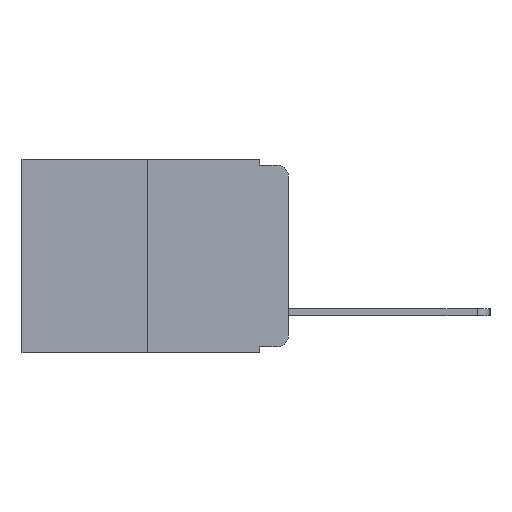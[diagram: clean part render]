
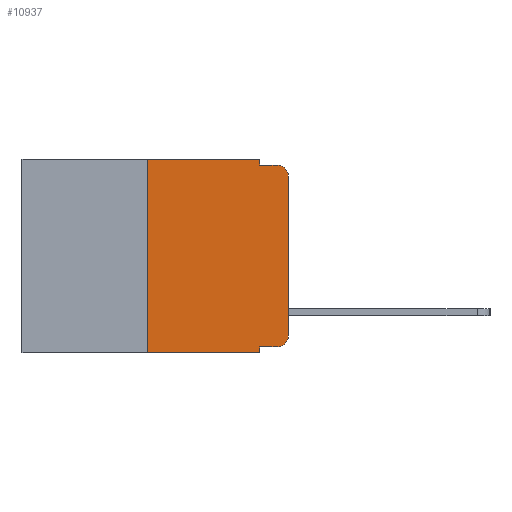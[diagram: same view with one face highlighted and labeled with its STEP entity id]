
A CAD part, left-side view. The second image highlights one B-rep face of the part: STEP entity #10937.
In plain terms, the highlighted planar face has unit normal (-1, 0, 0).
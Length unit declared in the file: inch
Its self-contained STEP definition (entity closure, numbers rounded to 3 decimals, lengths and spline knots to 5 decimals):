
#83 = EDGE_CURVE ( 'NONE', #4789, #15447, #14954, .T. ) ;
#96 = LINE ( 'NONE', #16927, #8019 ) ;
#361 = ORIENTED_EDGE ( 'NONE', *, *, #83, .F. ) ;
#401 = CARTESIAN_POINT ( 'NONE',  ( 0., 0.25, 0. ) ) ;
#1118 = ORIENTED_EDGE ( 'NONE', *, *, #17320, .T. ) ;
#1808 = LINE ( 'NONE', #2811, #13620 ) ;
#1845 = VECTOR ( 'NONE', #5247, 39.37008 ) ;
#2014 = DIRECTION ( 'NONE',  ( 0., 0., -1. ) ) ;
#2174 = VERTEX_POINT ( 'NONE', #8511 ) ;
#2244 = CARTESIAN_POINT ( 'NONE',  ( 0., 0.051, 0. ) ) ;
#2385 = EDGE_CURVE ( 'NONE', #12834, #7028, #96, .T. ) ;
#2429 = CIRCLE ( 'NONE', #7947, 0.02 ) ;
#2731 = DIRECTION ( 'NONE',  ( 0., 0., 1. ) ) ;
#2811 = CARTESIAN_POINT ( 'NONE',  ( 0., 0.051, 0. ) ) ;
#3052 = AXIS2_PLACEMENT_3D ( 'NONE', #17057, #8124, #18480 ) ;
#3173 = VECTOR ( 'NONE', #15278, 39.37008 ) ;
#3271 = EDGE_CURVE ( 'NONE', #6931, #4019, #18633, .T. ) ;
#3538 = VECTOR ( 'NONE', #13511, 39.37008 ) ;
#3826 = CARTESIAN_POINT ( 'NONE',  ( 0., 0.473, 0. ) ) ;
#4019 = VERTEX_POINT ( 'NONE', #2244 ) ;
#4202 = ORIENTED_EDGE ( 'NONE', *, *, #7983, .T. ) ;
#4789 = VERTEX_POINT ( 'NONE', #7397 ) ;
#5091 = FACE_OUTER_BOUND ( 'NONE', #15024, .T. ) ;
#5247 = DIRECTION ( 'NONE',  ( 0., -1., 0. ) ) ;
#5254 = DIRECTION ( 'NONE',  ( 0., 0., 1. ) ) ;
#5626 = ORIENTED_EDGE ( 'NONE', *, *, #8613, .T. ) ;
#6355 = ORIENTED_EDGE ( 'NONE', *, *, #9268, .F. ) ;
#6802 = VECTOR ( 'NONE', #17627, 39.37008 ) ;
#6863 = EDGE_CURVE ( 'NONE', #16658, #6931, #12802, .T. ) ;
#6915 = VECTOR ( 'NONE', #2014, 39.37008 ) ;
#6924 = DIRECTION ( 'NONE',  ( 1., 0., 0. ) ) ;
#6931 = VERTEX_POINT ( 'NONE', #8373 ) ;
#7028 = VERTEX_POINT ( 'NONE', #18915 ) ;
#7296 = CARTESIAN_POINT ( 'NONE',  ( 0., 0.051, -0.343 ) ) ;
#7326 = ORIENTED_EDGE ( 'NONE', *, *, #3271, .F. ) ;
#7397 = CARTESIAN_POINT ( 'NONE',  ( 0., 0.051, -0.333 ) ) ;
#7947 = AXIS2_PLACEMENT_3D ( 'NONE', #9153, #19458, #10696 ) ;
#7983 = EDGE_CURVE ( 'NONE', #16658, #15447, #14851, .T. ) ;
#8019 = VECTOR ( 'NONE', #2731, 39.37008 ) ;
#8124 = DIRECTION ( 'NONE',  ( -1., 0., 0. ) ) ;
#8261 = VECTOR ( 'NONE', #5254, 39.37008 ) ;
#8370 = PLANE ( 'NONE',  #16020 ) ;
#8373 = CARTESIAN_POINT ( 'NONE',  ( 0., 0.25, 0. ) ) ;
#8511 = CARTESIAN_POINT ( 'NONE',  ( 0., 0.051, -0.01 ) ) ;
#8613 = EDGE_CURVE ( 'NONE', #4789, #18017, #10090, .T. ) ;
#9153 = CARTESIAN_POINT ( 'NONE',  ( 0., 0.02, -0.03 ) ) ;
#9268 = EDGE_CURVE ( 'NONE', #4019, #2174, #1808, .T. ) ;
#9687 = VERTEX_POINT ( 'NONE', #11928 ) ;
#9906 = ORIENTED_EDGE ( 'NONE', *, *, #13094, .F. ) ;
#10090 = LINE ( 'NONE', #18586, #1845 ) ;
#10184 = CARTESIAN_POINT ( 'NONE',  ( 0., 0.25, -0.343 ) ) ;
#10696 = DIRECTION ( 'NONE',  ( 0., 0., -1. ) ) ;
#10937 = ADVANCED_FACE ( 'NONE', ( #5091 ), #8370, .F. ) ;
#11356 = ORIENTED_EDGE ( 'NONE', *, *, #6863, .F. ) ;
#11928 = CARTESIAN_POINT ( 'NONE',  ( 0., 0.02, -0.01 ) ) ;
#11991 = CARTESIAN_POINT ( 'NONE',  ( 0., 0.051, -0.01 ) ) ;
#12802 = LINE ( 'NONE', #401, #8261 ) ;
#12834 = VERTEX_POINT ( 'NONE', #15898 ) ;
#13094 = EDGE_CURVE ( 'NONE', #2174, #9687, #15618, .T. ) ;
#13451 = DIRECTION ( 'NONE',  ( 0., 0., -1. ) ) ;
#13511 = DIRECTION ( 'NONE',  ( 0., -1., 0. ) ) ;
#13620 = VECTOR ( 'NONE', #13451, 39.37008 ) ;
#13787 = CARTESIAN_POINT ( 'NONE',  ( 0., 0.473, -0.343 ) ) ;
#14493 = ORIENTED_EDGE ( 'NONE', *, *, #18327, .T. ) ;
#14851 = LINE ( 'NONE', #13787, #3173 ) ;
#14954 = LINE ( 'NONE', #18951, #6915 ) ;
#15024 = EDGE_LOOP ( 'NONE', ( #16441, #1118, #9906, #6355, #7326, #11356, #4202, #361, #5626, #14493 ) ) ;
#15278 = DIRECTION ( 'NONE',  ( 0., -1., 0. ) ) ;
#15447 = VERTEX_POINT ( 'NONE', #7296 ) ;
#15618 = LINE ( 'NONE', #11991, #3538 ) ;
#15898 = CARTESIAN_POINT ( 'NONE',  ( 0., 0., -0.313 ) ) ;
#16020 = AXIS2_PLACEMENT_3D ( 'NONE', #3826, #6924, #17368 ) ;
#16441 = ORIENTED_EDGE ( 'NONE', *, *, #2385, .T. ) ;
#16658 = VERTEX_POINT ( 'NONE', #10184 ) ;
#16927 = CARTESIAN_POINT ( 'NONE',  ( 0., 0., 0. ) ) ;
#17057 = CARTESIAN_POINT ( 'NONE',  ( 0., 0.02, -0.313 ) ) ;
#17320 = EDGE_CURVE ( 'NONE', #7028, #9687, #2429, .T. ) ;
#17368 = DIRECTION ( 'NONE',  ( 0., 0., -1. ) ) ;
#17606 = CARTESIAN_POINT ( 'NONE',  ( 0., 0.473, 0. ) ) ;
#17627 = DIRECTION ( 'NONE',  ( 0., -1., 0. ) ) ;
#17828 = CARTESIAN_POINT ( 'NONE',  ( 0., 0.02, -0.333 ) ) ;
#18017 = VERTEX_POINT ( 'NONE', #17828 ) ;
#18327 = EDGE_CURVE ( 'NONE', #18017, #12834, #19054, .T. ) ;
#18480 = DIRECTION ( 'NONE',  ( 0., 0., -1. ) ) ;
#18586 = CARTESIAN_POINT ( 'NONE',  ( 0., 0.051, -0.333 ) ) ;
#18633 = LINE ( 'NONE', #17606, #6802 ) ;
#18915 = CARTESIAN_POINT ( 'NONE',  ( 0., 0., -0.03 ) ) ;
#18951 = CARTESIAN_POINT ( 'NONE',  ( 0., 0.051, 0. ) ) ;
#19054 = CIRCLE ( 'NONE', #3052, 0.02 ) ;
#19458 = DIRECTION ( 'NONE',  ( -1., 0., 0. ) ) ;
